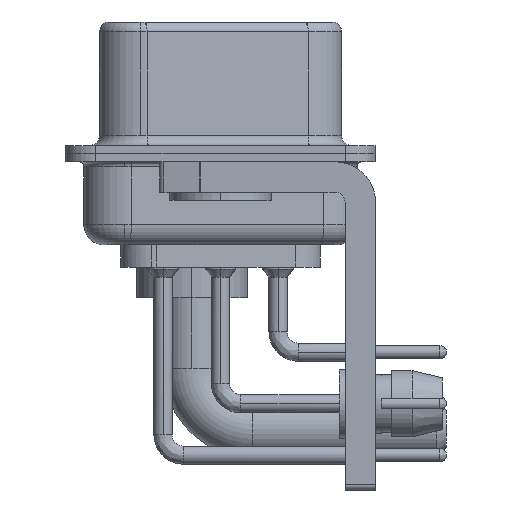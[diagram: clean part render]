
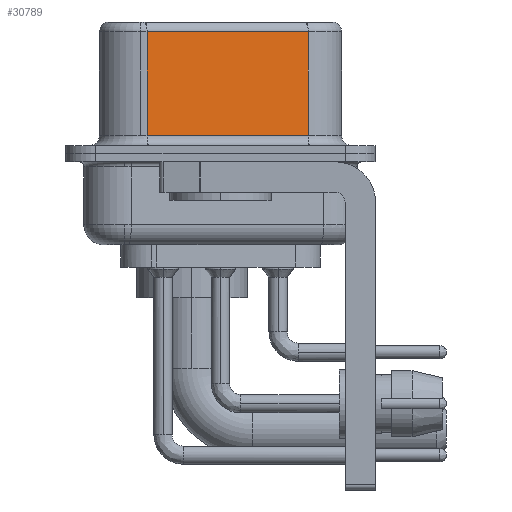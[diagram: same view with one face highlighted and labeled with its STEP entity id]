
A CAD part, left-side view. The second image highlights one B-rep face of the part: STEP entity #30789.
In plain terms, the highlighted planar face has unit normal (-0.985, -0.174, 0).
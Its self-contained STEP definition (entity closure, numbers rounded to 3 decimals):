
#1706 = DIRECTION ( 'NONE',  ( -0.174, 0.985, 0. ) ) ;
#2631 = VECTOR ( 'NONE', #31496, 1000. ) ;
#3789 = EDGE_CURVE ( 'NONE', #13792, #18143, #35318, .T. ) ;
#4363 = ORIENTED_EDGE ( 'NONE', *, *, #28302, .F. ) ;
#4912 = CARTESIAN_POINT ( 'NONE',  ( 3.73, 3.628, 6.02 ) ) ;
#6128 = DIRECTION ( 'NONE',  ( 0., 0., -1. ) ) ;
#7750 = PLANE ( 'NONE',  #8296 ) ;
#8296 = AXIS2_PLACEMENT_3D ( 'NONE', #17006, #29277, #1706 ) ;
#9185 = ORIENTED_EDGE ( 'NONE', *, *, #3789, .T. ) ;
#9778 = CARTESIAN_POINT ( 'NONE',  ( 5.132, -4.322, 6.02 ) ) ;
#10169 = EDGE_CURVE ( 'NONE', #18143, #20224, #17744, .T. ) ;
#12437 = EDGE_CURVE ( 'NONE', #37472, #13792, #37346, .T. ) ;
#13792 = VERTEX_POINT ( 'NONE', #4912 ) ;
#14631 = ORIENTED_EDGE ( 'NONE', *, *, #10169, .T. ) ;
#17006 = CARTESIAN_POINT ( 'NONE',  ( 5.132, -4.322, 6.52 ) ) ;
#17553 = VECTOR ( 'NONE', #34922, 1000. ) ;
#17744 = LINE ( 'NONE', #29996, #30849 ) ;
#18143 = VERTEX_POINT ( 'NONE', #39212 ) ;
#18155 = DIRECTION ( 'NONE',  ( 0.174, -0.985, 0. ) ) ;
#18281 = CARTESIAN_POINT ( 'NONE',  ( 5.132, -4.322, 0.9 ) ) ;
#18638 = LINE ( 'NONE', #30880, #37709 ) ;
#20224 = VERTEX_POINT ( 'NONE', #18281 ) ;
#22473 = ORIENTED_EDGE ( 'NONE', *, *, #12437, .T. ) ;
#23277 = CARTESIAN_POINT ( 'NONE',  ( 3.73, 3.628, 6.52 ) ) ;
#25790 = CARTESIAN_POINT ( 'NONE',  ( 5.132, -4.322, 6.02 ) ) ;
#28302 = EDGE_CURVE ( 'NONE', #37472, #20224, #18638, .T. ) ;
#29277 = DIRECTION ( 'NONE',  ( 0.985, 0.174, 0. ) ) ;
#29996 = CARTESIAN_POINT ( 'NONE',  ( 5.132, -4.322, 0.9 ) ) ;
#30789 = ADVANCED_FACE ( 'NONE', ( #35319 ), #7750, .F. ) ;
#30849 = VECTOR ( 'NONE', #18155, 1000. ) ;
#30880 = CARTESIAN_POINT ( 'NONE',  ( 5.132, -4.322, 6.52 ) ) ;
#31496 = DIRECTION ( 'NONE',  ( -0.174, 0.985, 0. ) ) ;
#33112 = EDGE_LOOP ( 'NONE', ( #4363, #22473, #9185, #14631 ) ) ;
#34922 = DIRECTION ( 'NONE',  ( 0., 0., -1. ) ) ;
#35318 = LINE ( 'NONE', #23277, #17553 ) ;
#35319 = FACE_OUTER_BOUND ( 'NONE', #33112, .T. ) ;
#37346 = LINE ( 'NONE', #9778, #2631 ) ;
#37472 = VERTEX_POINT ( 'NONE', #25790 ) ;
#37709 = VECTOR ( 'NONE', #6128, 1000. ) ;
#39212 = CARTESIAN_POINT ( 'NONE',  ( 3.73, 3.628, 0.9 ) ) ;
